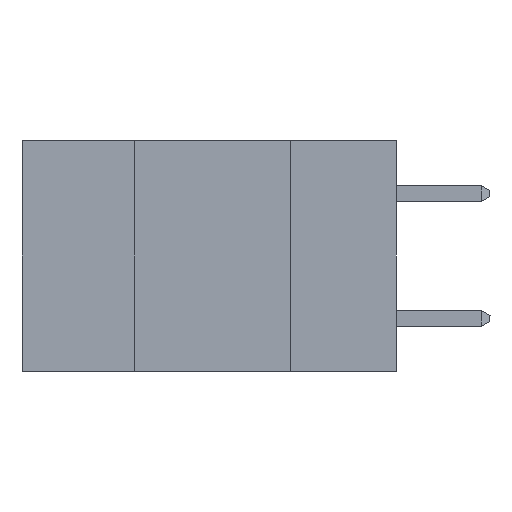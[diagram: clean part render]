
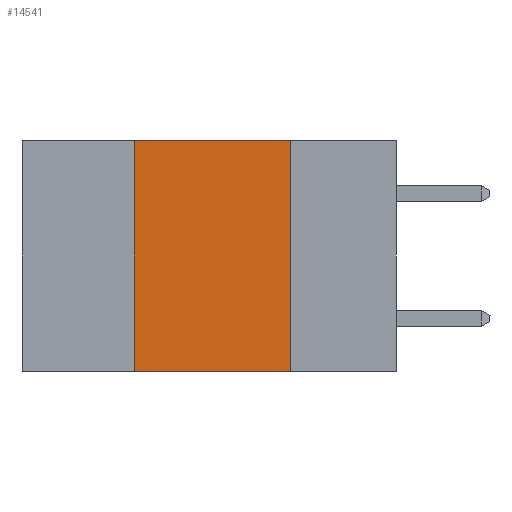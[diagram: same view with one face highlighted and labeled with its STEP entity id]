
A CAD part, left-side view. The second image highlights one B-rep face of the part: STEP entity #14541.
In plain terms, the highlighted planar face has unit normal (-1, 0, 0).
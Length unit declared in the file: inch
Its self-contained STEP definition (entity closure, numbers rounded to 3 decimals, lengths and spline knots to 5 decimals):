
#589 = CARTESIAN_POINT ( 'NONE',  ( 0., 0.6, 0. ) ) ;
#1104 = CARTESIAN_POINT ( 'NONE',  ( 0., 0.17, 0. ) ) ;
#1196 = FACE_OUTER_BOUND ( 'NONE', #14597, .T. ) ;
#1649 = ORIENTED_EDGE ( 'NONE', *, *, #13455, .F. ) ;
#2595 = LINE ( 'NONE', #589, #9411 ) ;
#2631 = CARTESIAN_POINT ( 'NONE',  ( 0., 0.6, -0.37 ) ) ;
#2886 = CARTESIAN_POINT ( 'NONE',  ( 0., 0.42, -0.37 ) ) ;
#2998 = CARTESIAN_POINT ( 'NONE',  ( 0., 0.42, -0.37 ) ) ;
#3030 = LINE ( 'NONE', #2631, #9842 ) ;
#3312 = DIRECTION ( 'NONE',  ( 0., -1., 0. ) ) ;
#3425 = CARTESIAN_POINT ( 'NONE',  ( 0., 0.42, 0. ) ) ;
#3564 = PLANE ( 'NONE',  #7500 ) ;
#4006 = DIRECTION ( 'NONE',  ( 0., -1., 0. ) ) ;
#4118 = VERTEX_POINT ( 'NONE', #1104 ) ;
#4397 = EDGE_CURVE ( 'NONE', #10000, #13281, #17163, .T. ) ;
#5684 = CARTESIAN_POINT ( 'NONE',  ( 0., 0.17, -0.37 ) ) ;
#6312 = DIRECTION ( 'NONE',  ( 0., 0., -1. ) ) ;
#7139 = EDGE_CURVE ( 'NONE', #13281, #4118, #2595, .T. ) ;
#7500 = AXIS2_PLACEMENT_3D ( 'NONE', #13041, #14424, #6312 ) ;
#9248 = CARTESIAN_POINT ( 'NONE',  ( 0., 0.17, -0.37 ) ) ;
#9411 = VECTOR ( 'NONE', #3312, 39.37008 ) ;
#9842 = VECTOR ( 'NONE', #4006, 39.37008 ) ;
#10000 = VERTEX_POINT ( 'NONE', #2886 ) ;
#10420 = ORIENTED_EDGE ( 'NONE', *, *, #10530, .T. ) ;
#10530 = EDGE_CURVE ( 'NONE', #10000, #11242, #3030, .T. ) ;
#10592 = VECTOR ( 'NONE', #15983, 39.37008 ) ;
#10818 = VECTOR ( 'NONE', #15208, 39.37008 ) ;
#11242 = VERTEX_POINT ( 'NONE', #5684 ) ;
#11443 = LINE ( 'NONE', #9248, #10592 ) ;
#13041 = CARTESIAN_POINT ( 'NONE',  ( 0., 0.6, 0. ) ) ;
#13281 = VERTEX_POINT ( 'NONE', #3425 ) ;
#13323 = ORIENTED_EDGE ( 'NONE', *, *, #7139, .F. ) ;
#13455 = EDGE_CURVE ( 'NONE', #4118, #11242, #11443, .T. ) ;
#14160 = ORIENTED_EDGE ( 'NONE', *, *, #4397, .F. ) ;
#14424 = DIRECTION ( 'NONE',  ( 1., 0., 0. ) ) ;
#14541 = ADVANCED_FACE ( 'NONE', ( #1196 ), #3564, .F. ) ;
#14597 = EDGE_LOOP ( 'NONE', ( #1649, #13323, #14160, #10420 ) ) ;
#15208 = DIRECTION ( 'NONE',  ( 0., 0., 1. ) ) ;
#15983 = DIRECTION ( 'NONE',  ( 0., 0., -1. ) ) ;
#17163 = LINE ( 'NONE', #2998, #10818 ) ;
